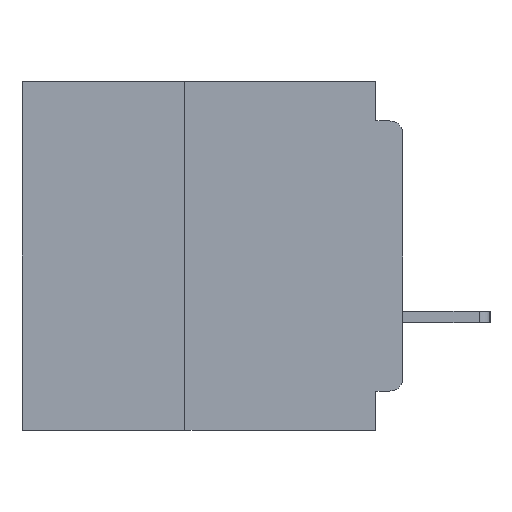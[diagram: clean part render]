
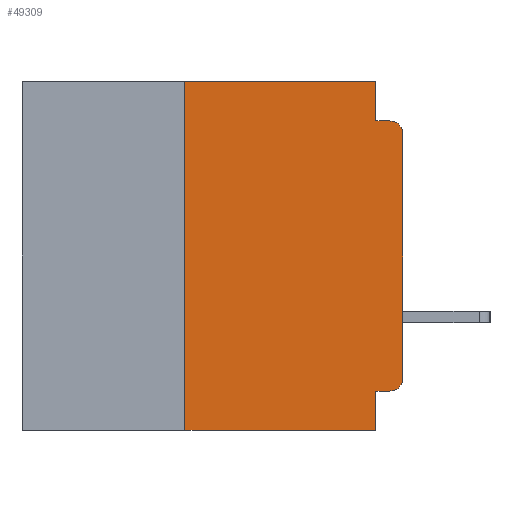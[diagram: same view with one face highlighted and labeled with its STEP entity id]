
A CAD part, left-side view. The second image highlights one B-rep face of the part: STEP entity #49309.
In plain terms, the highlighted planar face has unit normal (-1, 0, 0).
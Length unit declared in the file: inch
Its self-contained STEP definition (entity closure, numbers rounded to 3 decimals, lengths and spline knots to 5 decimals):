
#377 = FACE_OUTER_BOUND ( 'NONE', #34771, .T. ) ;
#785 = EDGE_CURVE ( 'NONE', #30458, #18773, #52736, .T. ) ;
#815 = VERTEX_POINT ( 'NONE', #24219 ) ;
#1392 = CARTESIAN_POINT ( 'NONE',  ( 0., 0.015, -0.045 ) ) ;
#2775 = VECTOR ( 'NONE', #45839, 39.37008 ) ;
#3504 = CARTESIAN_POINT ( 'NONE',  ( 0., 0.25, 0. ) ) ;
#3861 = CARTESIAN_POINT ( 'NONE',  ( 0., 0.031, -0.045 ) ) ;
#5030 = DIRECTION ( 'NONE',  ( 0., 1., 0. ) ) ;
#6984 = CIRCLE ( 'NONE', #59412, 0.015 ) ;
#7203 = PLANE ( 'NONE',  #51049 ) ;
#7500 = ORIENTED_EDGE ( 'NONE', *, *, #62225, .T. ) ;
#7702 = VERTEX_POINT ( 'NONE', #12008 ) ;
#9406 = VECTOR ( 'NONE', #37749, 39.37008 ) ;
#11324 = AXIS2_PLACEMENT_3D ( 'NONE', #15676, #15752, #15959 ) ;
#11395 = ORIENTED_EDGE ( 'NONE', *, *, #48589, .F. ) ;
#12008 = CARTESIAN_POINT ( 'NONE',  ( 0., 0.031, -0.355 ) ) ;
#12123 = DIRECTION ( 'NONE',  ( 1., 0., 0. ) ) ;
#12470 = CARTESIAN_POINT ( 'NONE',  ( 0., 0.031, -0.4 ) ) ;
#13049 = ORIENTED_EDGE ( 'NONE', *, *, #57681, .F. ) ;
#15420 = EDGE_CURVE ( 'NONE', #37235, #30458, #46735, .T. ) ;
#15508 = VECTOR ( 'NONE', #5030, 39.37008 ) ;
#15676 = CARTESIAN_POINT ( 'NONE',  ( 0., 0.015, -0.06 ) ) ;
#15752 = DIRECTION ( 'NONE',  ( -1., 0., 0. ) ) ;
#15959 = DIRECTION ( 'NONE',  ( 0., 0., -1. ) ) ;
#16709 = CARTESIAN_POINT ( 'NONE',  ( 0., 0.437, -0.4 ) ) ;
#16981 = LINE ( 'NONE', #38994, #54246 ) ;
#17424 = DIRECTION ( 'NONE',  ( 0., 0., -1. ) ) ;
#18420 = VECTOR ( 'NONE', #17424, 39.37008 ) ;
#18773 = VERTEX_POINT ( 'NONE', #1392 ) ;
#23155 = VERTEX_POINT ( 'NONE', #3504 ) ;
#23813 = ORIENTED_EDGE ( 'NONE', *, *, #15420, .T. ) ;
#23943 = DIRECTION ( 'NONE',  ( -1., 0., 0. ) ) ;
#24219 = CARTESIAN_POINT ( 'NONE',  ( 0., 0.031, 0. ) ) ;
#24381 = CARTESIAN_POINT ( 'NONE',  ( 0., 0., -0.06 ) ) ;
#24436 = VECTOR ( 'NONE', #38231, 39.37008 ) ;
#24583 = CARTESIAN_POINT ( 'NONE',  ( 0., 0., -0.355 ) ) ;
#27011 = DIRECTION ( 'NONE',  ( 0., -1., 0. ) ) ;
#27233 = LINE ( 'NONE', #36329, #49912 ) ;
#28545 = LINE ( 'NONE', #24583, #15508 ) ;
#30458 = VERTEX_POINT ( 'NONE', #24381 ) ;
#30636 = CARTESIAN_POINT ( 'NONE',  ( 0., 0.437, 0. ) ) ;
#33085 = EDGE_CURVE ( 'NONE', #34454, #23155, #16981, .T. ) ;
#33342 = CARTESIAN_POINT ( 'NONE',  ( 0., 0.031, 0. ) ) ;
#33425 = LINE ( 'NONE', #30636, #44777 ) ;
#34454 = VERTEX_POINT ( 'NONE', #45571 ) ;
#34771 = EDGE_LOOP ( 'NONE', ( #23813, #56083, #43783, #13049, #11395, #61528, #44864, #56488, #49981, #7500 ) ) ;
#36329 = CARTESIAN_POINT ( 'NONE',  ( 0., 0., -0.045 ) ) ;
#37235 = VERTEX_POINT ( 'NONE', #59372 ) ;
#37749 = DIRECTION ( 'NONE',  ( 0., 0., 1. ) ) ;
#38231 = DIRECTION ( 'NONE',  ( 0., 0., -1. ) ) ;
#38994 = CARTESIAN_POINT ( 'NONE',  ( 0., 0.25, -0.4 ) ) ;
#42208 = VERTEX_POINT ( 'NONE', #44096 ) ;
#43018 = CARTESIAN_POINT ( 'NONE',  ( 0., 0.031, -0.4 ) ) ;
#43783 = ORIENTED_EDGE ( 'NONE', *, *, #60222, .F. ) ;
#44096 = CARTESIAN_POINT ( 'NONE',  ( 0., 0.015, -0.355 ) ) ;
#44777 = VECTOR ( 'NONE', #59854, 39.37008 ) ;
#44864 = ORIENTED_EDGE ( 'NONE', *, *, #48629, .T. ) ;
#45133 = VERTEX_POINT ( 'NONE', #3861 ) ;
#45571 = CARTESIAN_POINT ( 'NONE',  ( 0., 0.25, -0.4 ) ) ;
#45839 = DIRECTION ( 'NONE',  ( 0., -1., 0. ) ) ;
#46181 = DIRECTION ( 'NONE',  ( 0., 0., -1. ) ) ;
#46735 = LINE ( 'NONE', #47437, #9406 ) ;
#47437 = CARTESIAN_POINT ( 'NONE',  ( 0., 0., 0. ) ) ;
#48589 = EDGE_CURVE ( 'NONE', #23155, #815, #33425, .T. ) ;
#48629 = EDGE_CURVE ( 'NONE', #34454, #49524, #54628, .T. ) ;
#49309 = ADVANCED_FACE ( 'NONE', ( #377 ), #7203, .F. ) ;
#49524 = VERTEX_POINT ( 'NONE', #43018 ) ;
#49912 = VECTOR ( 'NONE', #27011, 39.37008 ) ;
#49981 = ORIENTED_EDGE ( 'NONE', *, *, #50752, .F. ) ;
#50752 = EDGE_CURVE ( 'NONE', #42208, #7702, #28545, .T. ) ;
#50855 = CARTESIAN_POINT ( 'NONE',  ( 0., 0.437, 0. ) ) ;
#51049 = AXIS2_PLACEMENT_3D ( 'NONE', #50855, #12123, #46181 ) ;
#52736 = CIRCLE ( 'NONE', #11324, 0.015 ) ;
#52962 = CARTESIAN_POINT ( 'NONE',  ( 0., 0.015, -0.34 ) ) ;
#54246 = VECTOR ( 'NONE', #63140, 39.37008 ) ;
#54628 = LINE ( 'NONE', #16709, #2775 ) ;
#56083 = ORIENTED_EDGE ( 'NONE', *, *, #785, .T. ) ;
#56488 = ORIENTED_EDGE ( 'NONE', *, *, #62678, .F. ) ;
#57206 = LINE ( 'NONE', #12470, #18420 ) ;
#57681 = EDGE_CURVE ( 'NONE', #815, #45133, #63121, .T. ) ;
#57844 = DIRECTION ( 'NONE',  ( 0., 0., -1. ) ) ;
#59372 = CARTESIAN_POINT ( 'NONE',  ( 0., 0., -0.34 ) ) ;
#59412 = AXIS2_PLACEMENT_3D ( 'NONE', #52962, #23943, #57844 ) ;
#59854 = DIRECTION ( 'NONE',  ( 0., -1., 0. ) ) ;
#60222 = EDGE_CURVE ( 'NONE', #45133, #18773, #27233, .T. ) ;
#61528 = ORIENTED_EDGE ( 'NONE', *, *, #33085, .F. ) ;
#62225 = EDGE_CURVE ( 'NONE', #42208, #37235, #6984, .T. ) ;
#62678 = EDGE_CURVE ( 'NONE', #7702, #49524, #57206, .T. ) ;
#63121 = LINE ( 'NONE', #33342, #24436 ) ;
#63140 = DIRECTION ( 'NONE',  ( 0., 0., 1. ) ) ;
